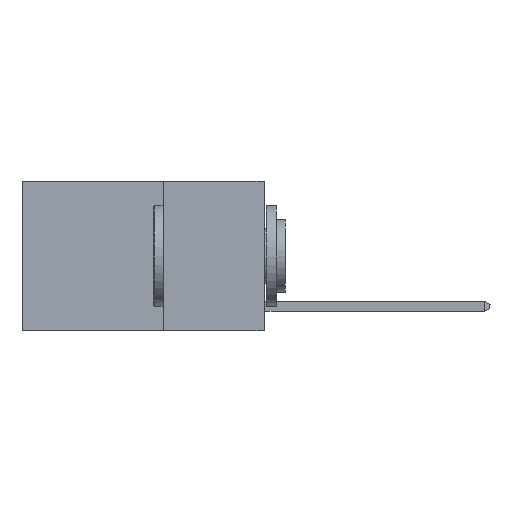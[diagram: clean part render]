
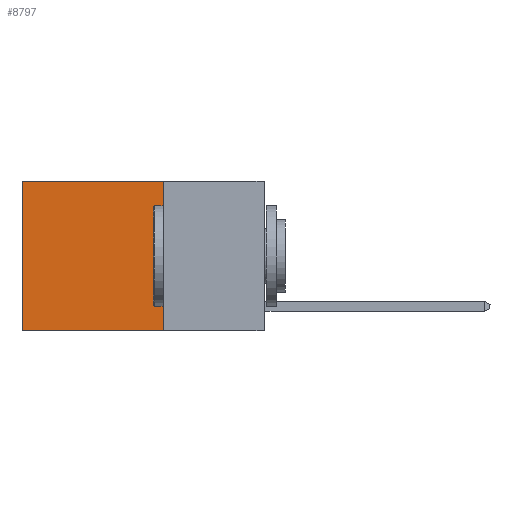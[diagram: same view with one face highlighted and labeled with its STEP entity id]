
A CAD part, left-side view. The second image highlights one B-rep face of the part: STEP entity #8797.
In plain terms, the highlighted planar face has unit normal (-1, 0, 0).
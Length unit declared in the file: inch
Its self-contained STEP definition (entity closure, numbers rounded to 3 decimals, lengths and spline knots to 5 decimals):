
#80 = CARTESIAN_POINT ( 'NONE',  ( 0.2625, 0.6, -0.37 ) ) ;
#963 = VERTEX_POINT ( 'NONE', #17854 ) ;
#1784 = CARTESIAN_POINT ( 'NONE',  ( 0.2625, 0.25, -0.37 ) ) ;
#3137 = CARTESIAN_POINT ( 'NONE',  ( 0.2625, 0.25, 0. ) ) ;
#3778 = VERTEX_POINT ( 'NONE', #80 ) ;
#4819 = EDGE_CURVE ( 'NONE', #963, #6937, #10337, .T. ) ;
#5147 = LINE ( 'NONE', #17228, #11400 ) ;
#5335 = DIRECTION ( 'NONE',  ( 0., 0., -1. ) ) ;
#6600 = CARTESIAN_POINT ( 'NONE',  ( 0.2625, 0.25, 0. ) ) ;
#6655 = CARTESIAN_POINT ( 'NONE',  ( 0.2625, 0.6, 0. ) ) ;
#6937 = VERTEX_POINT ( 'NONE', #1784 ) ;
#7931 = VECTOR ( 'NONE', #5335, 39.37008 ) ;
#8162 = ORIENTED_EDGE ( 'NONE', *, *, #23520, .F. ) ;
#8401 = ORIENTED_EDGE ( 'NONE', *, *, #10569, .T. ) ;
#8797 = ADVANCED_FACE ( 'NONE', ( #13675 ), #23271, .F. ) ;
#10056 = CARTESIAN_POINT ( 'NONE',  ( 0.2625, 0.25, -0.37 ) ) ;
#10337 = LINE ( 'NONE', #3137, #7931 ) ;
#10474 = EDGE_CURVE ( 'NONE', #963, #18687, #18519, .T. ) ;
#10569 = EDGE_CURVE ( 'NONE', #18687, #3778, #5147, .T. ) ;
#11400 = VECTOR ( 'NONE', #12353, 39.37008 ) ;
#12353 = DIRECTION ( 'NONE',  ( 0., 0., -1. ) ) ;
#13675 = FACE_OUTER_BOUND ( 'NONE', #20264, .T. ) ;
#15095 = LINE ( 'NONE', #10056, #15904 ) ;
#15851 = AXIS2_PLACEMENT_3D ( 'NONE', #6600, #30657, #28280 ) ;
#15904 = VECTOR ( 'NONE', #24525, 39.37008 ) ;
#16307 = CARTESIAN_POINT ( 'NONE',  ( 0.2625, 0.25, 0. ) ) ;
#17228 = CARTESIAN_POINT ( 'NONE',  ( 0.2625, 0.6, 0. ) ) ;
#17668 = ORIENTED_EDGE ( 'NONE', *, *, #4819, .F. ) ;
#17854 = CARTESIAN_POINT ( 'NONE',  ( 0.2625, 0.25, 0. ) ) ;
#18437 = VECTOR ( 'NONE', #26214, 39.37008 ) ;
#18519 = LINE ( 'NONE', #16307, #18437 ) ;
#18687 = VERTEX_POINT ( 'NONE', #6655 ) ;
#20264 = EDGE_LOOP ( 'NONE', ( #8401, #8162, #17668, #26572 ) ) ;
#23271 = PLANE ( 'NONE',  #15851 ) ;
#23520 = EDGE_CURVE ( 'NONE', #6937, #3778, #15095, .T. ) ;
#24525 = DIRECTION ( 'NONE',  ( 0., 1., 0. ) ) ;
#26214 = DIRECTION ( 'NONE',  ( 0., 1., 0. ) ) ;
#26572 = ORIENTED_EDGE ( 'NONE', *, *, #10474, .T. ) ;
#28280 = DIRECTION ( 'NONE',  ( 0., 0., -1. ) ) ;
#30657 = DIRECTION ( 'NONE',  ( 1., 0., 0. ) ) ;
